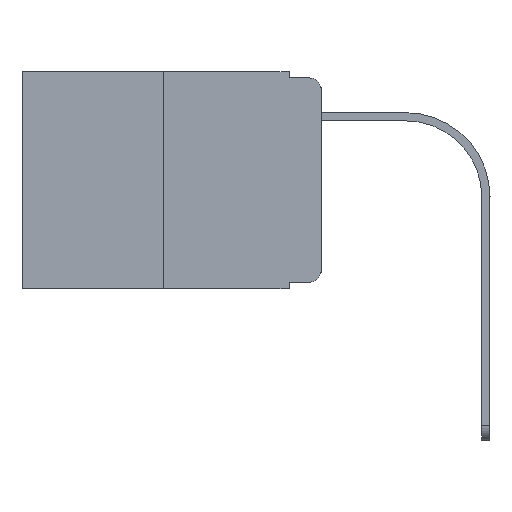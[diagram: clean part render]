
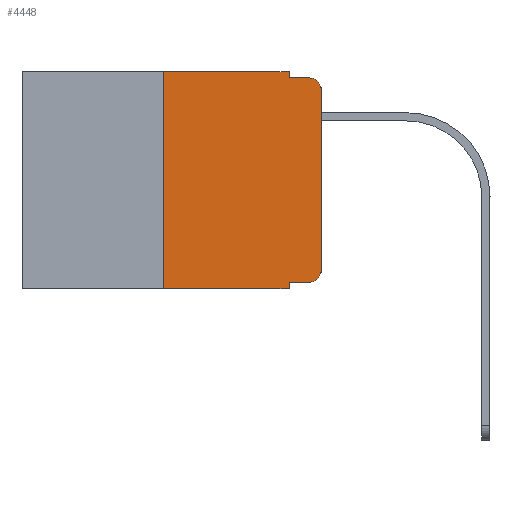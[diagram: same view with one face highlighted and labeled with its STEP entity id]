
A CAD part, left-side view. The second image highlights one B-rep face of the part: STEP entity #4448.
In plain terms, the highlighted planar face has unit normal (-1, 0, 0).
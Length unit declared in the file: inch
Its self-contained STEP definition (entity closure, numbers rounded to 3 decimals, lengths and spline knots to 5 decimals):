
#255 = CARTESIAN_POINT ( 'NONE',  ( 0., 0.25, 0. ) ) ;
#437 = DIRECTION ( 'NONE',  ( 0., 0., -1. ) ) ;
#485 = EDGE_CURVE ( 'NONE', #2650, #11300, #3883, .T. ) ;
#486 = ORIENTED_EDGE ( 'NONE', *, *, #9004, .T. ) ;
#491 = VECTOR ( 'NONE', #3848, 39.37008 ) ;
#600 = VERTEX_POINT ( 'NONE', #2032 ) ;
#641 = CARTESIAN_POINT ( 'NONE',  ( 0., 0.25, 0. ) ) ;
#956 = CARTESIAN_POINT ( 'NONE',  ( 0., 0.051, 0. ) ) ;
#1017 = DIRECTION ( 'NONE',  ( 0., 0., -1. ) ) ;
#1067 = ORIENTED_EDGE ( 'NONE', *, *, #8053, .T. ) ;
#1224 = CARTESIAN_POINT ( 'NONE',  ( 0., 0.25, -0.343 ) ) ;
#1240 = CARTESIAN_POINT ( 'NONE',  ( 0., 0.02, -0.01 ) ) ;
#1333 = CARTESIAN_POINT ( 'NONE',  ( 0., 0.02, -0.313 ) ) ;
#1445 = VERTEX_POINT ( 'NONE', #7387 ) ;
#1460 = ORIENTED_EDGE ( 'NONE', *, *, #7252, .F. ) ;
#1472 = LINE ( 'NONE', #3224, #6628 ) ;
#1549 = DIRECTION ( 'NONE',  ( 0., 0., 1. ) ) ;
#1787 = LINE ( 'NONE', #6345, #4727 ) ;
#1848 = LINE ( 'NONE', #956, #2652 ) ;
#1971 = ORIENTED_EDGE ( 'NONE', *, *, #485, .T. ) ;
#2032 = CARTESIAN_POINT ( 'NONE',  ( 0., 0.051, -0.333 ) ) ;
#2081 = VECTOR ( 'NONE', #7787, 39.37008 ) ;
#2121 = VECTOR ( 'NONE', #6247, 39.37008 ) ;
#2577 = EDGE_CURVE ( 'NONE', #600, #9304, #1787, .T. ) ;
#2613 = ORIENTED_EDGE ( 'NONE', *, *, #7104, .F. ) ;
#2650 = VERTEX_POINT ( 'NONE', #5596 ) ;
#2652 = VECTOR ( 'NONE', #1017, 39.37008 ) ;
#2664 = CIRCLE ( 'NONE', #6013, 0.02 ) ;
#2693 = CARTESIAN_POINT ( 'NONE',  ( 0., 0.051, 0. ) ) ;
#3072 = DIRECTION ( 'NONE',  ( 0., 0., 1. ) ) ;
#3159 = ORIENTED_EDGE ( 'NONE', *, *, #3264, .F. ) ;
#3224 = CARTESIAN_POINT ( 'NONE',  ( 0., 0.473, -0.343 ) ) ;
#3264 = EDGE_CURVE ( 'NONE', #6004, #1445, #10404, .T. ) ;
#3341 = FACE_OUTER_BOUND ( 'NONE', #5511, .T. ) ;
#3784 = EDGE_CURVE ( 'NONE', #7245, #10679, #9269, .T. ) ;
#3848 = DIRECTION ( 'NONE',  ( 0., -1., 0. ) ) ;
#3883 = LINE ( 'NONE', #4682, #4898 ) ;
#4219 = AXIS2_PLACEMENT_3D ( 'NONE', #1333, #11198, #437 ) ;
#4448 = ADVANCED_FACE ( 'NONE', ( #3341 ), #9759, .F. ) ;
#4643 = CARTESIAN_POINT ( 'NONE',  ( 0., 0.051, -0.01 ) ) ;
#4682 = CARTESIAN_POINT ( 'NONE',  ( 0., 0., 0. ) ) ;
#4726 = LINE ( 'NONE', #2693, #2121 ) ;
#4727 = VECTOR ( 'NONE', #7342, 39.37008 ) ;
#4763 = EDGE_CURVE ( 'NONE', #1445, #7245, #1848, .T. ) ;
#4783 = CIRCLE ( 'NONE', #4219, 0.02 ) ;
#4898 = VECTOR ( 'NONE', #3072, 39.37008 ) ;
#4911 = CARTESIAN_POINT ( 'NONE',  ( 0., 0.02, -0.333 ) ) ;
#5043 = EDGE_CURVE ( 'NONE', #11300, #10679, #2664, .T. ) ;
#5247 = CARTESIAN_POINT ( 'NONE',  ( 0., 0.02, -0.03 ) ) ;
#5447 = AXIS2_PLACEMENT_3D ( 'NONE', #6896, #9579, #11521 ) ;
#5511 = EDGE_LOOP ( 'NONE', ( #1971, #9801, #5761, #10410, #3159, #2613, #1067, #1460, #5577, #486 ) ) ;
#5577 = ORIENTED_EDGE ( 'NONE', *, *, #2577, .T. ) ;
#5596 = CARTESIAN_POINT ( 'NONE',  ( 0., 0., -0.313 ) ) ;
#5636 = VERTEX_POINT ( 'NONE', #1224 ) ;
#5761 = ORIENTED_EDGE ( 'NONE', *, *, #3784, .F. ) ;
#6004 = VERTEX_POINT ( 'NONE', #255 ) ;
#6013 = AXIS2_PLACEMENT_3D ( 'NONE', #5247, #11345, #6181 ) ;
#6102 = CARTESIAN_POINT ( 'NONE',  ( 0., 0.473, 0. ) ) ;
#6181 = DIRECTION ( 'NONE',  ( 0., 0., -1. ) ) ;
#6247 = DIRECTION ( 'NONE',  ( 0., 0., -1. ) ) ;
#6345 = CARTESIAN_POINT ( 'NONE',  ( 0., 0.051, -0.333 ) ) ;
#6628 = VECTOR ( 'NONE', #7752, 39.37008 ) ;
#6896 = CARTESIAN_POINT ( 'NONE',  ( 0., 0.473, 0. ) ) ;
#7104 = EDGE_CURVE ( 'NONE', #5636, #6004, #8712, .T. ) ;
#7245 = VERTEX_POINT ( 'NONE', #7343 ) ;
#7252 = EDGE_CURVE ( 'NONE', #600, #10350, #4726, .T. ) ;
#7342 = DIRECTION ( 'NONE',  ( 0., -1., 0. ) ) ;
#7343 = CARTESIAN_POINT ( 'NONE',  ( 0., 0.051, -0.01 ) ) ;
#7387 = CARTESIAN_POINT ( 'NONE',  ( 0., 0.051, 0. ) ) ;
#7752 = DIRECTION ( 'NONE',  ( 0., -1., 0. ) ) ;
#7787 = DIRECTION ( 'NONE',  ( 0., -1., 0. ) ) ;
#8053 = EDGE_CURVE ( 'NONE', #5636, #10350, #1472, .T. ) ;
#8283 = CARTESIAN_POINT ( 'NONE',  ( 0., 0.051, -0.343 ) ) ;
#8712 = LINE ( 'NONE', #641, #9415 ) ;
#9004 = EDGE_CURVE ( 'NONE', #9304, #2650, #4783, .T. ) ;
#9200 = CARTESIAN_POINT ( 'NONE',  ( 0., 0., -0.03 ) ) ;
#9269 = LINE ( 'NONE', #4643, #491 ) ;
#9304 = VERTEX_POINT ( 'NONE', #4911 ) ;
#9415 = VECTOR ( 'NONE', #1549, 39.37008 ) ;
#9579 = DIRECTION ( 'NONE',  ( 1., 0., 0. ) ) ;
#9759 = PLANE ( 'NONE',  #5447 ) ;
#9801 = ORIENTED_EDGE ( 'NONE', *, *, #5043, .T. ) ;
#10350 = VERTEX_POINT ( 'NONE', #8283 ) ;
#10404 = LINE ( 'NONE', #6102, #2081 ) ;
#10410 = ORIENTED_EDGE ( 'NONE', *, *, #4763, .F. ) ;
#10679 = VERTEX_POINT ( 'NONE', #1240 ) ;
#11198 = DIRECTION ( 'NONE',  ( -1., 0., 0. ) ) ;
#11300 = VERTEX_POINT ( 'NONE', #9200 ) ;
#11345 = DIRECTION ( 'NONE',  ( -1., 0., 0. ) ) ;
#11521 = DIRECTION ( 'NONE',  ( 0., 0., -1. ) ) ;
